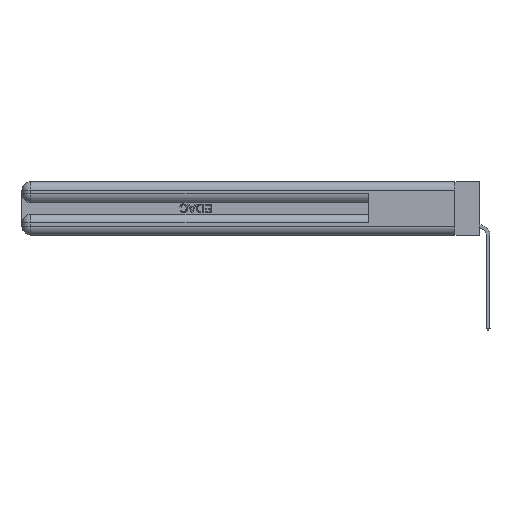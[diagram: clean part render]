
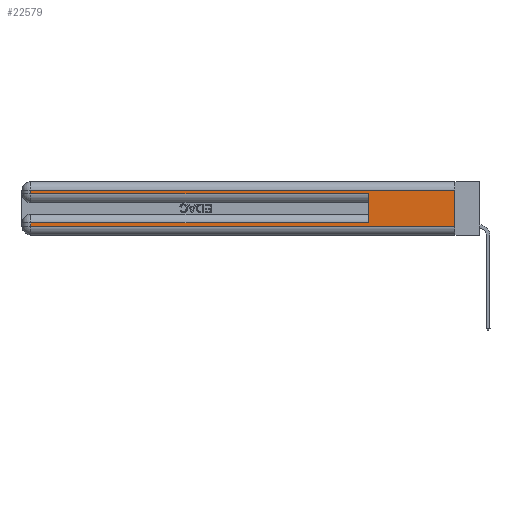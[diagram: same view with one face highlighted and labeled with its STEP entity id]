
A CAD part, left-side view. The second image highlights one B-rep face of the part: STEP entity #22579.
In plain terms, the highlighted planar face has unit normal (-1, 0, 0).
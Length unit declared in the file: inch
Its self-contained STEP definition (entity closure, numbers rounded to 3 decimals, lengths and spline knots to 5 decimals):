
#199 = CARTESIAN_POINT ( 'NONE',  ( 0., 2.94, 0.285 ) ) ;
#740 = LINE ( 'NONE', #1171, #5983 ) ;
#953 = ORIENTED_EDGE ( 'NONE', *, *, #7546, .T. ) ;
#972 = ORIENTED_EDGE ( 'NONE', *, *, #27298, .T. ) ;
#1171 = CARTESIAN_POINT ( 'NONE',  ( 0., 0.6, 0.145 ) ) ;
#2125 = VERTEX_POINT ( 'NONE', #17404 ) ;
#2614 = VECTOR ( 'NONE', #27346, 39.37008 ) ;
#2935 = LINE ( 'NONE', #27155, #10122 ) ;
#2999 = CARTESIAN_POINT ( 'NONE',  ( 0., 2.94, 0.37 ) ) ;
#3234 = CARTESIAN_POINT ( 'NONE',  ( 0., 0., 0.37 ) ) ;
#3237 = VECTOR ( 'NONE', #16531, 39.37008 ) ;
#3791 = LINE ( 'NONE', #14448, #8455 ) ;
#3812 = LINE ( 'NONE', #10415, #17654 ) ;
#4402 = VERTEX_POINT ( 'NONE', #17426 ) ;
#5862 = AXIS2_PLACEMENT_3D ( 'NONE', #16788, #20829, #12175 ) ;
#5983 = VECTOR ( 'NONE', #22830, 39.37008 ) ;
#6537 = ORIENTED_EDGE ( 'NONE', *, *, #13505, .T. ) ;
#7155 = CARTESIAN_POINT ( 'NONE',  ( 0., 0.6, 0.285 ) ) ;
#7498 = EDGE_CURVE ( 'NONE', #17546, #15866, #740, .T. ) ;
#7546 = EDGE_CURVE ( 'NONE', #2125, #13283, #2935, .T. ) ;
#7727 = LINE ( 'NONE', #3234, #16423 ) ;
#8037 = FACE_OUTER_BOUND ( 'NONE', #12080, .T. ) ;
#8455 = VECTOR ( 'NONE', #23235, 39.37008 ) ;
#9763 = VERTEX_POINT ( 'NONE', #10705 ) ;
#9965 = DIRECTION ( 'NONE',  ( 0., 1., 0. ) ) ;
#10009 = CARTESIAN_POINT ( 'NONE',  ( 0., 2.94, 0.37 ) ) ;
#10122 = VECTOR ( 'NONE', #9965, 39.37008 ) ;
#10415 = CARTESIAN_POINT ( 'NONE',  ( 0., 0., 0.06 ) ) ;
#10705 = CARTESIAN_POINT ( 'NONE',  ( 0., 2.94, 0.085 ) ) ;
#11891 = CARTESIAN_POINT ( 'NONE',  ( 0., 0., 0.085 ) ) ;
#12080 = EDGE_LOOP ( 'NONE', ( #13054, #953, #12631, #6537, #15071, #15263, #972, #17814 ) ) ;
#12175 = DIRECTION ( 'NONE',  ( 0., 0., -1. ) ) ;
#12631 = ORIENTED_EDGE ( 'NONE', *, *, #18707, .T. ) ;
#13054 = ORIENTED_EDGE ( 'NONE', *, *, #19517, .F. ) ;
#13283 = VERTEX_POINT ( 'NONE', #14340 ) ;
#13505 = EDGE_CURVE ( 'NONE', #18378, #15866, #3791, .T. ) ;
#14050 = LINE ( 'NONE', #11891, #2614 ) ;
#14175 = EDGE_CURVE ( 'NONE', #15373, #4402, #3812, .T. ) ;
#14340 = CARTESIAN_POINT ( 'NONE',  ( 0., 2.94, 0.31 ) ) ;
#14448 = CARTESIAN_POINT ( 'NONE',  ( 0., 0., 0.285 ) ) ;
#15071 = ORIENTED_EDGE ( 'NONE', *, *, #7498, .F. ) ;
#15263 = ORIENTED_EDGE ( 'NONE', *, *, #19804, .T. ) ;
#15373 = VERTEX_POINT ( 'NONE', #27384 ) ;
#15866 = VERTEX_POINT ( 'NONE', #7155 ) ;
#16423 = VECTOR ( 'NONE', #24833, 39.37008 ) ;
#16531 = DIRECTION ( 'NONE',  ( 0., 0., -1. ) ) ;
#16788 = CARTESIAN_POINT ( 'NONE',  ( 0., 0., 0.37 ) ) ;
#17060 = DIRECTION ( 'NONE',  ( 0., 0., -1. ) ) ;
#17404 = CARTESIAN_POINT ( 'NONE',  ( 0., 0., 0.31 ) ) ;
#17426 = CARTESIAN_POINT ( 'NONE',  ( 0., 0., 0.06 ) ) ;
#17546 = VERTEX_POINT ( 'NONE', #20934 ) ;
#17654 = VECTOR ( 'NONE', #25847, 39.37008 ) ;
#17814 = ORIENTED_EDGE ( 'NONE', *, *, #14175, .T. ) ;
#18378 = VERTEX_POINT ( 'NONE', #199 ) ;
#18674 = LINE ( 'NONE', #2999, #3237 ) ;
#18707 = EDGE_CURVE ( 'NONE', #13283, #18378, #19206, .T. ) ;
#19206 = LINE ( 'NONE', #10009, #20992 ) ;
#19517 = EDGE_CURVE ( 'NONE', #2125, #4402, #7727, .T. ) ;
#19804 = EDGE_CURVE ( 'NONE', #17546, #9763, #14050, .T. ) ;
#20829 = DIRECTION ( 'NONE',  ( 1., 0., 0. ) ) ;
#20934 = CARTESIAN_POINT ( 'NONE',  ( 0., 0.6, 0.085 ) ) ;
#20992 = VECTOR ( 'NONE', #17060, 39.37008 ) ;
#22579 = ADVANCED_FACE ( 'NONE', ( #8037 ), #25311, .F. ) ;
#22830 = DIRECTION ( 'NONE',  ( 0., 0., 1. ) ) ;
#23235 = DIRECTION ( 'NONE',  ( 0., -1., 0. ) ) ;
#24833 = DIRECTION ( 'NONE',  ( 0., 0., -1. ) ) ;
#25311 = PLANE ( 'NONE',  #5862 ) ;
#25847 = DIRECTION ( 'NONE',  ( 0., -1., 0. ) ) ;
#27155 = CARTESIAN_POINT ( 'NONE',  ( 0., 0., 0.31 ) ) ;
#27298 = EDGE_CURVE ( 'NONE', #9763, #15373, #18674, .T. ) ;
#27346 = DIRECTION ( 'NONE',  ( 0., 1., 0. ) ) ;
#27384 = CARTESIAN_POINT ( 'NONE',  ( 0., 2.94, 0.06 ) ) ;
